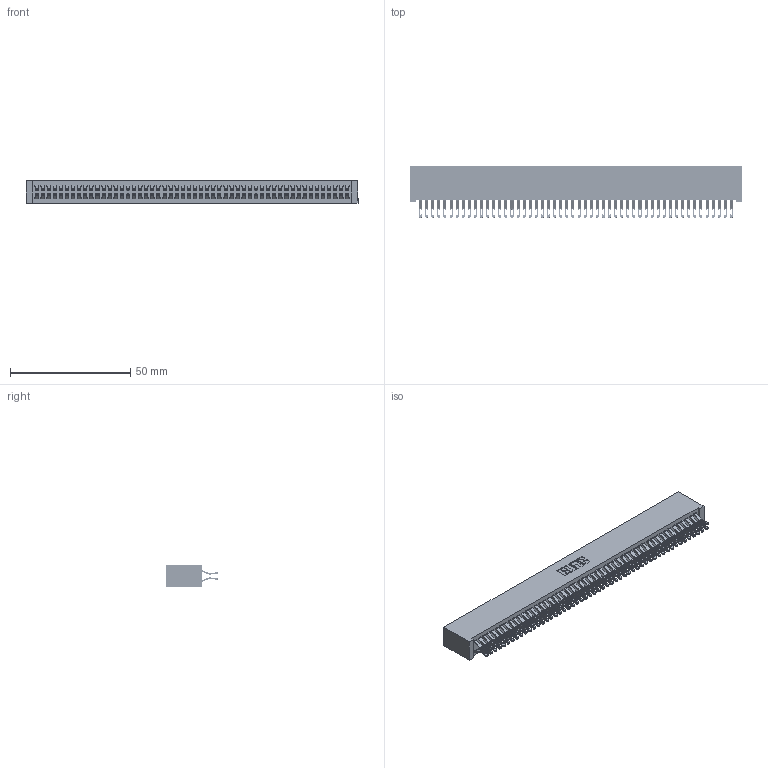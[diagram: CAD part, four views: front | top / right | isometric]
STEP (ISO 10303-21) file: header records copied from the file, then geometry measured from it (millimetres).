
FILE_DESCRIPTION (( 'STEP AP203' ), '1' );
FILE_NAME ('392-104-555-201.STEP', '2018-08-18T19:45:09', ( '' ), ( '' ), 'SwSTEP 2.0', 'SolidWorks 2016', '' );
FILE_SCHEMA (( 'CONFIG_CONTROL_DESIGN' ));
Length unit declared in the file: inch
Products named in the file (3): 342 Part_Lugless; 345-292-001_555 Tail; 392-104-555-201
Assembly tree (105 placements, depth 2):
  392-104-555-201
    342 Part_Lugless
    345-292-001_555 Tail  x104
Bounding box: 138.33 x 21.47 x 9.4 mm (x, y, z)
Volume: 13204.6 mm3; surface area: 23192.8 mm2
Topology: 105 solids, 105 shells, 6134 faces, 19307 edges, 12870 vertices
Faces by surface type: plane 3598, cylinder 2536
Entity records: 32077 total; most frequent: CARTESIAN_POINT 5336, ORIENTED_EDGE 5242, DIRECTION 4505, EDGE_CURVE 2621, LINE 2481, VECTOR 2481, VERTEX_POINT 1746, AXIS2_PLACEMENT_3D 1012
